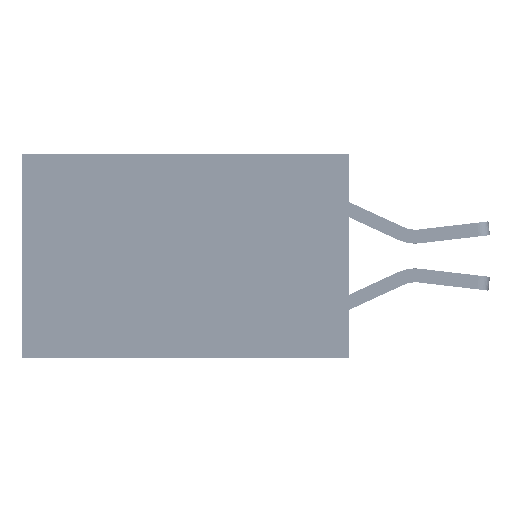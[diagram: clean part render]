
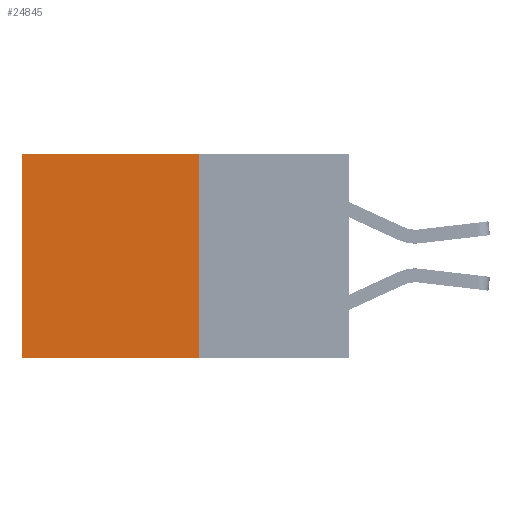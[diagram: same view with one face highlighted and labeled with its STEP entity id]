
A CAD part, left-side view. The second image highlights one B-rep face of the part: STEP entity #24845.
In plain terms, the highlighted planar face has unit normal (-1, 0, 0).
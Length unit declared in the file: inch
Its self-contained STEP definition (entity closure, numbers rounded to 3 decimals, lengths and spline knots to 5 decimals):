
#707 = VECTOR ( 'NONE', #5544, 39.37008 ) ;
#1167 = CARTESIAN_POINT ( 'NONE',  ( 0.277, 0.27, 0. ) ) ;
#1433 = VERTEX_POINT ( 'NONE', #9771 ) ;
#4235 = CARTESIAN_POINT ( 'NONE',  ( 0.277, 0.59, -0.37 ) ) ;
#4943 = VERTEX_POINT ( 'NONE', #23592 ) ;
#5431 = EDGE_CURVE ( 'NONE', #16506, #4943, #8974, .T. ) ;
#5544 = DIRECTION ( 'NONE',  ( 0., 0., -1. ) ) ;
#7750 = FACE_OUTER_BOUND ( 'NONE', #20807, .T. ) ;
#8372 = ORIENTED_EDGE ( 'NONE', *, *, #24316, .T. ) ;
#8974 = LINE ( 'NONE', #1167, #29684 ) ;
#9771 = CARTESIAN_POINT ( 'NONE',  ( 0.277, 0.27, -0.37 ) ) ;
#10345 = VECTOR ( 'NONE', #17744, 39.37008 ) ;
#11989 = ORIENTED_EDGE ( 'NONE', *, *, #29200, .F. ) ;
#12627 = ORIENTED_EDGE ( 'NONE', *, *, #5431, .T. ) ;
#14399 = DIRECTION ( 'NONE',  ( 1., 0., 0. ) ) ;
#15014 = DIRECTION ( 'NONE',  ( 0., 1., 0. ) ) ;
#15156 = LINE ( 'NONE', #21651, #707 ) ;
#16276 = ORIENTED_EDGE ( 'NONE', *, *, #29760, .F. ) ;
#16506 = VERTEX_POINT ( 'NONE', #20506 ) ;
#17521 = LINE ( 'NONE', #4235, #10345 ) ;
#17744 = DIRECTION ( 'NONE',  ( 0., 0., -1. ) ) ;
#20326 = AXIS2_PLACEMENT_3D ( 'NONE', #22592, #14399, #28010 ) ;
#20506 = CARTESIAN_POINT ( 'NONE',  ( 0.277, 0.27, 0. ) ) ;
#20807 = EDGE_LOOP ( 'NONE', ( #8372, #11989, #16276, #12627 ) ) ;
#21651 = CARTESIAN_POINT ( 'NONE',  ( 0.277, 0.27, -0.37 ) ) ;
#22592 = CARTESIAN_POINT ( 'NONE',  ( 0.277, 0.27, -0.37 ) ) ;
#22725 = CARTESIAN_POINT ( 'NONE',  ( 0.277, 0.27, -0.37 ) ) ;
#23592 = CARTESIAN_POINT ( 'NONE',  ( 0.277, 0.59, 0. ) ) ;
#24316 = EDGE_CURVE ( 'NONE', #4943, #31373, #17521, .T. ) ;
#24845 = ADVANCED_FACE ( 'NONE', ( #7750 ), #25307, .F. ) ;
#25113 = CARTESIAN_POINT ( 'NONE',  ( 0.277, 0.59, -0.37 ) ) ;
#25307 = PLANE ( 'NONE',  #20326 ) ;
#25330 = VECTOR ( 'NONE', #30796, 39.37008 ) ;
#28010 = DIRECTION ( 'NONE',  ( 0., 0., -1. ) ) ;
#29200 = EDGE_CURVE ( 'NONE', #1433, #31373, #32432, .T. ) ;
#29684 = VECTOR ( 'NONE', #15014, 39.37008 ) ;
#29760 = EDGE_CURVE ( 'NONE', #16506, #1433, #15156, .T. ) ;
#30796 = DIRECTION ( 'NONE',  ( 0., 1., 0. ) ) ;
#31373 = VERTEX_POINT ( 'NONE', #25113 ) ;
#32432 = LINE ( 'NONE', #22725, #25330 ) ;
